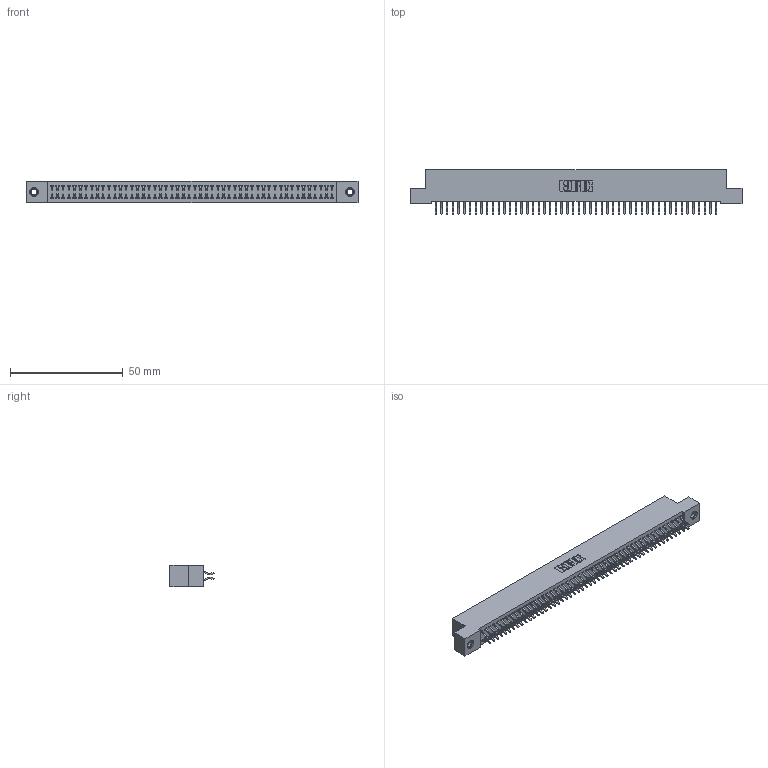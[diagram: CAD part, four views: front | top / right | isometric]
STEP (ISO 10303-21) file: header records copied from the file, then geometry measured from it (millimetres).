
FILE_DESCRIPTION (( 'STEP AP203' ), '1' );
FILE_NAME ('342-100-556-207.STEP', '2018-08-14T04:50:54', ( '' ), ( '' ), 'SwSTEP 2.0', 'SolidWorks 2016', '' );
FILE_SCHEMA (( 'CONFIG_CONTROL_DESIGN' ));
Length unit declared in the file: inch
Products named in the file (4): 345-292-001_556 Tail; 345-250-001_345-250-005-103; 342-100-556-207; 342 Part_TI
Assembly tree (103 placements, depth 2):
  342-100-556-207
    342 Part_TI
    345-292-001_556 Tail  x100
    345-250-001_345-250-005-103  x2
Bounding box: 147.32 x 19.58 x 9.4 mm (x, y, z)
Volume: 13259.3 mm3; surface area: 21708.8 mm2
Topology: 103 solids, 103 shells, 5970 faces, 17735 edges, 11682 vertices
Faces by surface type: plane 4098, cylinder 1856, cone 12, torus 4
Entity records: 32406 total; most frequent: CARTESIAN_POINT 5357, ORIENTED_EDGE 5274, DIRECTION 4583, EDGE_CURVE 2637, LINE 2481, VECTOR 2481, VERTEX_POINT 1752, AXIS2_PLACEMENT_3D 1051
